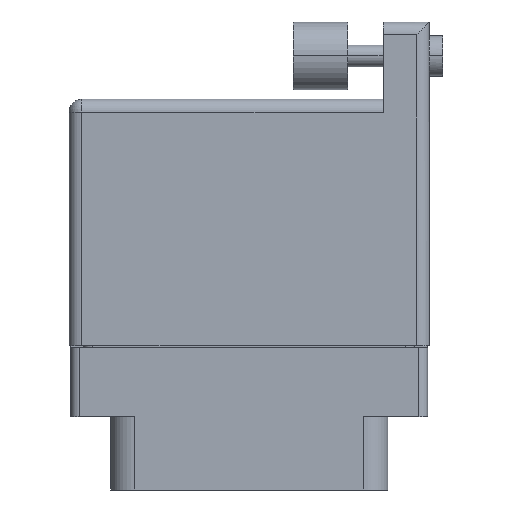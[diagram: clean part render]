
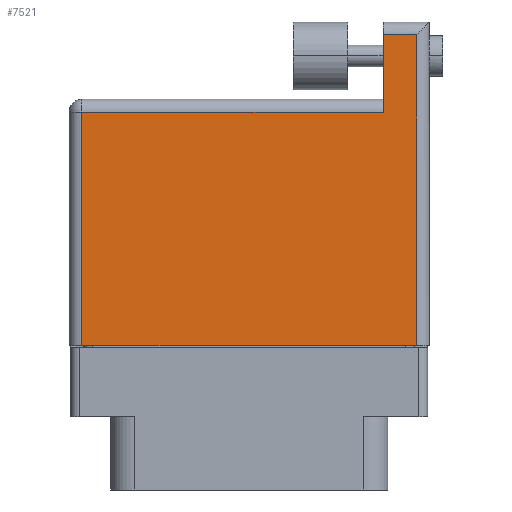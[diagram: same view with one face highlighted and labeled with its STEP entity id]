
A CAD part, front view. The second image highlights one B-rep face of the part: STEP entity #7521.
In plain terms, the highlighted face is planar.
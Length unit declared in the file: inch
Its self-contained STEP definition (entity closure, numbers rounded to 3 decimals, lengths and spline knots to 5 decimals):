
#132 = VECTOR ( 'NONE', #28744, 39.37008 ) ;
#189 = DIRECTION ( 'NONE',  ( 0., -1., 0. ) ) ;
#1440 = VERTEX_POINT ( 'NONE', #24942 ) ;
#2252 = ORIENTED_EDGE ( 'NONE', *, *, #18990, .T. ) ;
#2456 = EDGE_CURVE ( 'NONE', #29705, #7505, #2500, .T. ) ;
#2500 = LINE ( 'NONE', #21282, #22838 ) ;
#2826 = VECTOR ( 'NONE', #17487, 39.37008 ) ;
#3010 = CARTESIAN_POINT ( 'NONE',  ( -0.6155, 0.759, 0.3575 ) ) ;
#3272 = LINE ( 'NONE', #26700, #4132 ) ;
#3900 = VERTEX_POINT ( 'NONE', #8646 ) ;
#4132 = VECTOR ( 'NONE', #21767, 39.37008 ) ;
#4330 = DIRECTION ( 'NONE',  ( 0., 0., -1. ) ) ;
#4506 = EDGE_LOOP ( 'NONE', ( #28568, #21626, #2252, #12122, #10796, #22143 ) ) ;
#6128 = DIRECTION ( 'NONE',  ( 0., -1., 0. ) ) ;
#6649 = FACE_OUTER_BOUND ( 'NONE', #4506, .T. ) ;
#7174 = EDGE_CURVE ( 'NONE', #13418, #3900, #24362, .T. ) ;
#7505 = VERTEX_POINT ( 'NONE', #14175 ) ;
#7521 = ADVANCED_FACE ( 'NONE', ( #6649 ), #16035, .F. ) ;
#8646 = CARTESIAN_POINT ( 'NONE',  ( 0.6155, 1.043, 0.3575 ) ) ;
#9504 = CARTESIAN_POINT ( 'NONE',  ( 0.4925, 1.043, 0.3575 ) ) ;
#10064 = DIRECTION ( 'NONE',  ( 0., 1., 0. ) ) ;
#10321 = EDGE_CURVE ( 'NONE', #7505, #13418, #3272, .T. ) ;
#10796 = ORIENTED_EDGE ( 'NONE', *, *, #29826, .T. ) ;
#11056 = CARTESIAN_POINT ( 'NONE',  ( 0.4925, 1.09, 0.3575 ) ) ;
#11149 = EDGE_CURVE ( 'NONE', #1440, #16859, #12897, .T. ) ;
#12122 = ORIENTED_EDGE ( 'NONE', *, *, #11149, .T. ) ;
#12897 = LINE ( 'NONE', #11056, #13031 ) ;
#13031 = VECTOR ( 'NONE', #6128, 39.37008 ) ;
#13418 = VERTEX_POINT ( 'NONE', #17611 ) ;
#13700 = CARTESIAN_POINT ( 'NONE',  ( 0.4925, 0.759, 0.3575 ) ) ;
#13719 = DIRECTION ( 'NONE',  ( -1., 0., 0. ) ) ;
#14175 = CARTESIAN_POINT ( 'NONE',  ( -0.6155, -0.1, 0.3575 ) ) ;
#15619 = LINE ( 'NONE', #29502, #2826 ) ;
#16035 = PLANE ( 'NONE',  #24649 ) ;
#16859 = VERTEX_POINT ( 'NONE', #13700 ) ;
#17487 = DIRECTION ( 'NONE',  ( -1., 0., 0. ) ) ;
#17611 = CARTESIAN_POINT ( 'NONE',  ( 0.6155, -0.1, 0.3575 ) ) ;
#18990 = EDGE_CURVE ( 'NONE', #3900, #1440, #26116, .T. ) ;
#19699 = VECTOR ( 'NONE', #10064, 39.37008 ) ;
#21282 = CARTESIAN_POINT ( 'NONE',  ( -0.6155, -0.1, 0.3575 ) ) ;
#21626 = ORIENTED_EDGE ( 'NONE', *, *, #7174, .T. ) ;
#21767 = DIRECTION ( 'NONE',  ( 1., 0., 0. ) ) ;
#22143 = ORIENTED_EDGE ( 'NONE', *, *, #2456, .T. ) ;
#22838 = VECTOR ( 'NONE', #189, 39.37008 ) ;
#24208 = CARTESIAN_POINT ( 'NONE',  ( 0.6155, 1.09, 0.3575 ) ) ;
#24362 = LINE ( 'NONE', #24208, #19699 ) ;
#24649 = AXIS2_PLACEMENT_3D ( 'NONE', #25437, #4330, #13719 ) ;
#24942 = CARTESIAN_POINT ( 'NONE',  ( 0.4925, 1.043, 0.3575 ) ) ;
#25437 = CARTESIAN_POINT ( 'NONE',  ( -0.6625, 0.806, 0.3575 ) ) ;
#26116 = LINE ( 'NONE', #9504, #132 ) ;
#26700 = CARTESIAN_POINT ( 'NONE',  ( -0.6625, -0.1, 0.3575 ) ) ;
#28568 = ORIENTED_EDGE ( 'NONE', *, *, #10321, .T. ) ;
#28744 = DIRECTION ( 'NONE',  ( -1., 0., 0. ) ) ;
#29502 = CARTESIAN_POINT ( 'NONE',  ( -0.6625, 0.759, 0.3575 ) ) ;
#29705 = VERTEX_POINT ( 'NONE', #3010 ) ;
#29826 = EDGE_CURVE ( 'NONE', #16859, #29705, #15619, .T. ) ;
